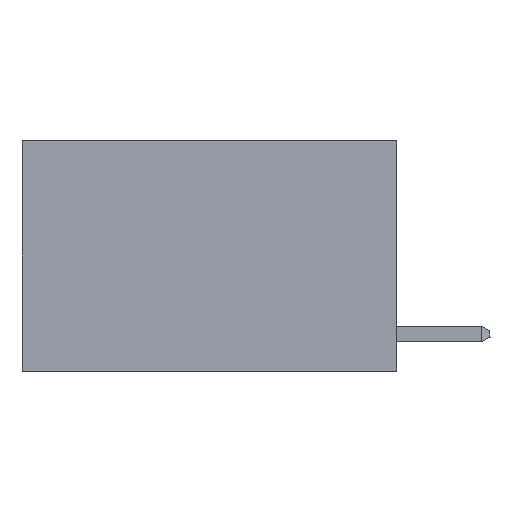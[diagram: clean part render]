
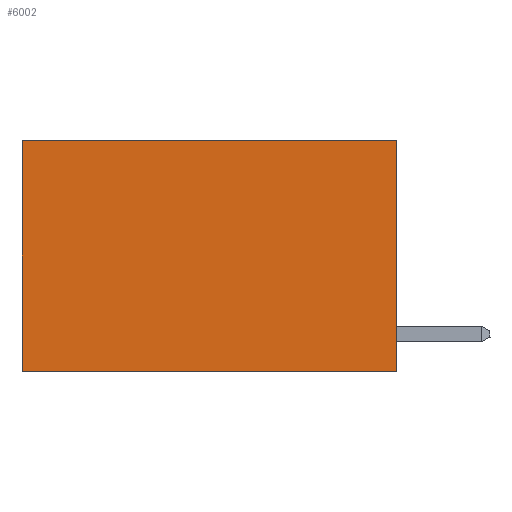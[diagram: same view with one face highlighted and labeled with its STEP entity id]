
A CAD part, left-side view. The second image highlights one B-rep face of the part: STEP entity #6002.
In plain terms, the highlighted planar face has unit normal (-1, 0, 0).
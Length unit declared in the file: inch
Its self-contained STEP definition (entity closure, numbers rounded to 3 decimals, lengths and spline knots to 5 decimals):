
#159 = CARTESIAN_POINT ( 'NONE',  ( 0.2625, 0.6, 0. ) ) ;
#206 = EDGE_CURVE ( 'NONE', #10717, #8925, #3263, .T. ) ;
#329 = VECTOR ( 'NONE', #10100, 39.37008 ) ;
#1011 = VERTEX_POINT ( 'NONE', #6160 ) ;
#3263 = LINE ( 'NONE', #4668, #11146 ) ;
#3476 = VECTOR ( 'NONE', #18718, 39.37008 ) ;
#3885 = ORIENTED_EDGE ( 'NONE', *, *, #206, .F. ) ;
#4668 = CARTESIAN_POINT ( 'NONE',  ( 0.2625, 0., -0.37 ) ) ;
#4706 = LINE ( 'NONE', #8521, #329 ) ;
#5877 = AXIS2_PLACEMENT_3D ( 'NONE', #18501, #9145, #20050 ) ;
#6002 = ADVANCED_FACE ( 'NONE', ( #8713 ), #7548, .F. ) ;
#6160 = CARTESIAN_POINT ( 'NONE',  ( 0.2625, 0., 0. ) ) ;
#6295 = CARTESIAN_POINT ( 'NONE',  ( 0.2625, 0., 0. ) ) ;
#6601 = CARTESIAN_POINT ( 'NONE',  ( 0.2625, 0., -0.37 ) ) ;
#7548 = PLANE ( 'NONE',  #5877 ) ;
#7728 = ORIENTED_EDGE ( 'NONE', *, *, #18299, .T. ) ;
#7776 = CARTESIAN_POINT ( 'NONE',  ( 0.2625, 0.6, 0. ) ) ;
#8202 = EDGE_CURVE ( 'NONE', #1011, #10717, #4706, .T. ) ;
#8521 = CARTESIAN_POINT ( 'NONE',  ( 0.2625, 0., 0. ) ) ;
#8713 = FACE_OUTER_BOUND ( 'NONE', #8975, .T. ) ;
#8925 = VERTEX_POINT ( 'NONE', #19120 ) ;
#8975 = EDGE_LOOP ( 'NONE', ( #17208, #3885, #11839, #7728 ) ) ;
#9145 = DIRECTION ( 'NONE',  ( 1., 0., 0. ) ) ;
#9966 = LINE ( 'NONE', #6295, #17806 ) ;
#10100 = DIRECTION ( 'NONE',  ( 0., 0., -1. ) ) ;
#10717 = VERTEX_POINT ( 'NONE', #6601 ) ;
#11146 = VECTOR ( 'NONE', #14439, 39.37008 ) ;
#11839 = ORIENTED_EDGE ( 'NONE', *, *, #8202, .F. ) ;
#14439 = DIRECTION ( 'NONE',  ( 0., 1., 0. ) ) ;
#15124 = EDGE_CURVE ( 'NONE', #19603, #8925, #15566, .T. ) ;
#15566 = LINE ( 'NONE', #7776, #3476 ) ;
#17208 = ORIENTED_EDGE ( 'NONE', *, *, #15124, .T. ) ;
#17806 = VECTOR ( 'NONE', #18824, 39.37008 ) ;
#18299 = EDGE_CURVE ( 'NONE', #1011, #19603, #9966, .T. ) ;
#18501 = CARTESIAN_POINT ( 'NONE',  ( 0.2625, 0., 0. ) ) ;
#18718 = DIRECTION ( 'NONE',  ( 0., 0., -1. ) ) ;
#18824 = DIRECTION ( 'NONE',  ( 0., 1., 0. ) ) ;
#19120 = CARTESIAN_POINT ( 'NONE',  ( 0.2625, 0.6, -0.37 ) ) ;
#19603 = VERTEX_POINT ( 'NONE', #159 ) ;
#20050 = DIRECTION ( 'NONE',  ( 0., 0., -1. ) ) ;
